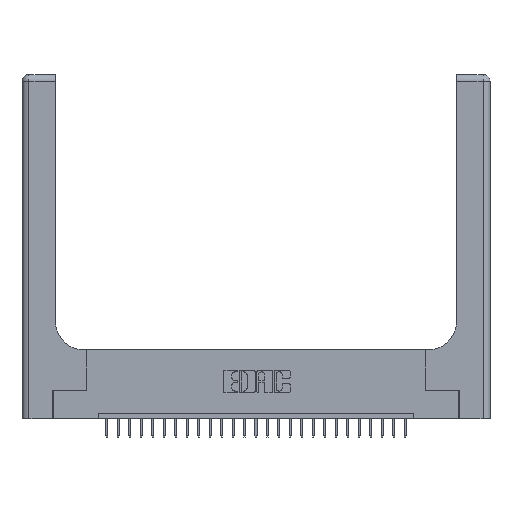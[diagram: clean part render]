
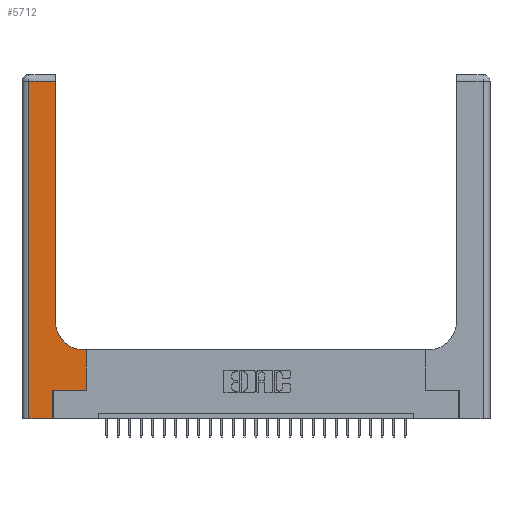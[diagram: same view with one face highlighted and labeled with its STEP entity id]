
A CAD part, top view. The second image highlights one B-rep face of the part: STEP entity #5712.
In plain terms, the highlighted planar face has unit normal (0, 0, 1).
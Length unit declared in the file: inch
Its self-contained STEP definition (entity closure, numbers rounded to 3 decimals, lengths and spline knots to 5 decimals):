
#308 = VERTEX_POINT ( 'NONE', #20649 ) ;
#578 = VERTEX_POINT ( 'NONE', #10025 ) ;
#1718 = CARTESIAN_POINT ( 'NONE',  ( 0.2915, 0.6, 0.37 ) ) ;
#2287 = VECTOR ( 'NONE', #8968, 39.37008 ) ;
#2736 = ORIENTED_EDGE ( 'NONE', *, *, #14785, .T. ) ;
#3447 = VERTEX_POINT ( 'NONE', #23218 ) ;
#3649 = EDGE_CURVE ( 'NONE', #308, #3447, #8162, .T. ) ;
#3873 = DIRECTION ( 'NONE',  ( 0., 0., -1. ) ) ;
#3876 = EDGE_LOOP ( 'NONE', ( #13962, #7123, #13675, #16584, #18419, #2736, #13955, #10823, #27448 ) ) ;
#4117 = LINE ( 'NONE', #9869, #16770 ) ;
#5712 = ADVANCED_FACE ( 'NONE', ( #17353 ), #16622, .F. ) ;
#5805 = VERTEX_POINT ( 'NONE', #21418 ) ;
#6667 = CARTESIAN_POINT ( 'NONE',  ( 0.269, 0., 0.37 ) ) ;
#6786 = DIRECTION ( 'NONE',  ( 1., 0., 0. ) ) ;
#6949 = VECTOR ( 'NONE', #26849, 39.37008 ) ;
#7123 = ORIENTED_EDGE ( 'NONE', *, *, #8360, .T. ) ;
#7598 = DIRECTION ( 'NONE',  ( 0., 1., 0. ) ) ;
#7602 = LINE ( 'NONE', #1718, #9287 ) ;
#7858 = EDGE_CURVE ( 'NONE', #8208, #5805, #24900, .T. ) ;
#8162 = CIRCLE ( 'NONE', #10769, 0.25 ) ;
#8208 = VERTEX_POINT ( 'NONE', #12823 ) ;
#8360 = EDGE_CURVE ( 'NONE', #16837, #8208, #14923, .T. ) ;
#8806 = CARTESIAN_POINT ( 'NONE',  ( 0.269, 0.25, 0.37 ) ) ;
#8876 = CARTESIAN_POINT ( 'NONE',  ( 0.06, 3., 0.37 ) ) ;
#8968 = DIRECTION ( 'NONE',  ( 0., -1., 0. ) ) ;
#9029 = CARTESIAN_POINT ( 'NONE',  ( 0.5415, 0.85, 0.37 ) ) ;
#9287 = VECTOR ( 'NONE', #14223, 39.37008 ) ;
#9859 = CARTESIAN_POINT ( 'NONE',  ( 0., 2.94, 0.37 ) ) ;
#9869 = CARTESIAN_POINT ( 'NONE',  ( 0.5585, 0.25, 0.37 ) ) ;
#10025 = CARTESIAN_POINT ( 'NONE',  ( 0.5585, 0.6, 0.37 ) ) ;
#10047 = CARTESIAN_POINT ( 'NONE',  ( 0., 0., 0.37 ) ) ;
#10140 = LINE ( 'NONE', #6667, #14133 ) ;
#10141 = DIRECTION ( 'NONE',  ( 0., 1., 0. ) ) ;
#10318 = EDGE_CURVE ( 'NONE', #27430, #578, #4117, .T. ) ;
#10769 = AXIS2_PLACEMENT_3D ( 'NONE', #9029, #11189, #6786 ) ;
#10823 = ORIENTED_EDGE ( 'NONE', *, *, #18216, .T. ) ;
#11189 = DIRECTION ( 'NONE',  ( 0., 0., -1. ) ) ;
#11422 = CARTESIAN_POINT ( 'NONE',  ( 0.269, 0.25, 0.37 ) ) ;
#11884 = CARTESIAN_POINT ( 'NONE',  ( 0.5585, 0.25, 0.37 ) ) ;
#12753 = AXIS2_PLACEMENT_3D ( 'NONE', #14324, #3873, #20879 ) ;
#12823 = CARTESIAN_POINT ( 'NONE',  ( 0.06, 2.94, 0.37 ) ) ;
#13240 = EDGE_CURVE ( 'NONE', #24084, #16742, #10140, .T. ) ;
#13675 = ORIENTED_EDGE ( 'NONE', *, *, #7858, .T. ) ;
#13955 = ORIENTED_EDGE ( 'NONE', *, *, #10318, .T. ) ;
#13962 = ORIENTED_EDGE ( 'NONE', *, *, #26856, .T. ) ;
#14133 = VECTOR ( 'NONE', #14407, 39.37008 ) ;
#14223 = DIRECTION ( 'NONE',  ( -1., 0., 0. ) ) ;
#14324 = CARTESIAN_POINT ( 'NONE',  ( 0., 3., 0.37 ) ) ;
#14407 = DIRECTION ( 'NONE',  ( 0., 1., 0. ) ) ;
#14785 = EDGE_CURVE ( 'NONE', #16742, #27430, #16371, .T. ) ;
#14923 = LINE ( 'NONE', #9859, #6949 ) ;
#16157 = VECTOR ( 'NONE', #10141, 39.37008 ) ;
#16371 = LINE ( 'NONE', #8806, #24308 ) ;
#16450 = CARTESIAN_POINT ( 'NONE',  ( 0.2915, 3., 0.37 ) ) ;
#16584 = ORIENTED_EDGE ( 'NONE', *, *, #26872, .T. ) ;
#16622 = PLANE ( 'NONE',  #12753 ) ;
#16742 = VERTEX_POINT ( 'NONE', #11422 ) ;
#16770 = VECTOR ( 'NONE', #7598, 39.37008 ) ;
#16837 = VERTEX_POINT ( 'NONE', #24556 ) ;
#17149 = VECTOR ( 'NONE', #24876, 39.37008 ) ;
#17353 = FACE_OUTER_BOUND ( 'NONE', #3876, .T. ) ;
#17460 = CARTESIAN_POINT ( 'NONE',  ( 0.269, 0., 0.37 ) ) ;
#18216 = EDGE_CURVE ( 'NONE', #578, #308, #7602, .T. ) ;
#18419 = ORIENTED_EDGE ( 'NONE', *, *, #13240, .T. ) ;
#20649 = CARTESIAN_POINT ( 'NONE',  ( 0.5415, 0.6, 0.37 ) ) ;
#20879 = DIRECTION ( 'NONE',  ( -1., 0., 0. ) ) ;
#21321 = DIRECTION ( 'NONE',  ( 1., 0., 0. ) ) ;
#21418 = CARTESIAN_POINT ( 'NONE',  ( 0.06, 0., 0.37 ) ) ;
#21771 = LINE ( 'NONE', #16450, #16157 ) ;
#22780 = LINE ( 'NONE', #10047, #17149 ) ;
#23218 = CARTESIAN_POINT ( 'NONE',  ( 0.2915, 0.85, 0.37 ) ) ;
#24084 = VERTEX_POINT ( 'NONE', #17460 ) ;
#24308 = VECTOR ( 'NONE', #21321, 39.37008 ) ;
#24556 = CARTESIAN_POINT ( 'NONE',  ( 0.2915, 2.94, 0.37 ) ) ;
#24876 = DIRECTION ( 'NONE',  ( 1., 0., 0. ) ) ;
#24900 = LINE ( 'NONE', #8876, #2287 ) ;
#26849 = DIRECTION ( 'NONE',  ( -1., 0., 0. ) ) ;
#26856 = EDGE_CURVE ( 'NONE', #3447, #16837, #21771, .T. ) ;
#26872 = EDGE_CURVE ( 'NONE', #5805, #24084, #22780, .T. ) ;
#27430 = VERTEX_POINT ( 'NONE', #11884 ) ;
#27448 = ORIENTED_EDGE ( 'NONE', *, *, #3649, .T. ) ;
